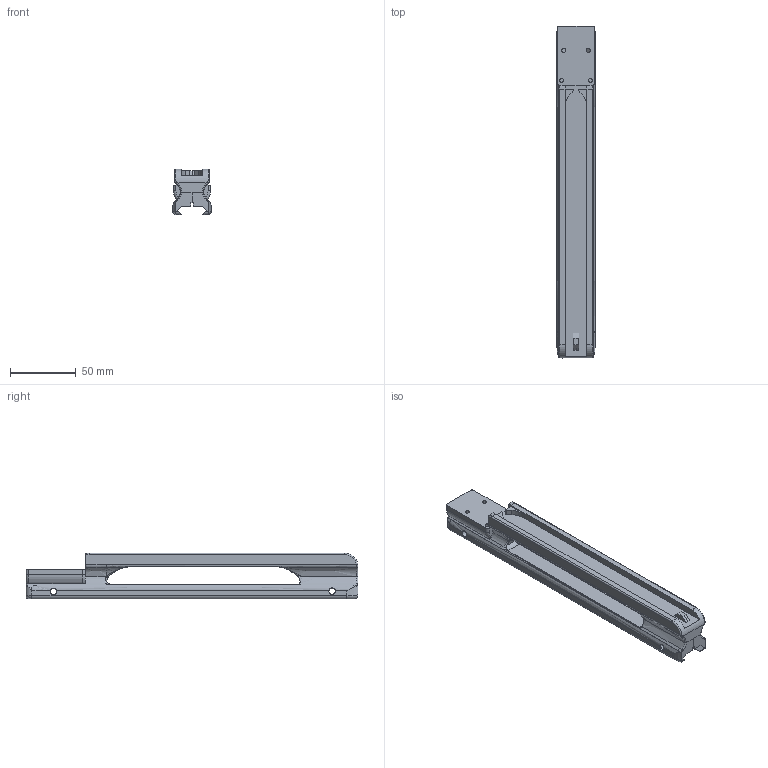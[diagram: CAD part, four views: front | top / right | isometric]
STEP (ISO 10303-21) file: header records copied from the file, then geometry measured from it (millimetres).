
FILE_DESCRIPTION(/* description */ (''),/* implementation_level */ '2;1');
FILE_NAME(/* name */ 'SG22 Carry Handle RMR Release.step',/* time_stamp */ '2021-03-18T08:57:38-06:00',/* author */ (''),/* organization */ (''),/* preprocessor_version */ 'ST-DEVELOPER v18.1',/* originating_system */ 'Autodesk Translation Framework v9.10.0.1330',/* authorisation */ '');
FILE_SCHEMA (('AUTOMOTIVE_DESIGN { 1 0 10303 214 3 1 1 }'));
Length unit declared in the file: millimetre
Products named in the file (1): Brace V2
Bounding box: 28.96 x 252.07 x 34.52 mm (x, y, z)
Volume: 115193.3 mm3; surface area: 43892.1 mm2
Topology: 1 solids, 1 shells, 289 faces, 826 edges, 530 vertices
Faces by surface type: plane 158, bspline 62, cylinder 51, torus 10, sphere 8
Full cylindrical faces by diameter (mm): 3 x4, 5 x4, 5.004 x2
Entity records: 11732 total; most frequent: CARTESIAN_POINT 4595, ORIENTED_EDGE 1652, DIRECTION 1235, EDGE_CURVE 826, VERTEX_POINT 530, LINE 453, VECTOR 453, AXIS2_PLACEMENT_3D 391
